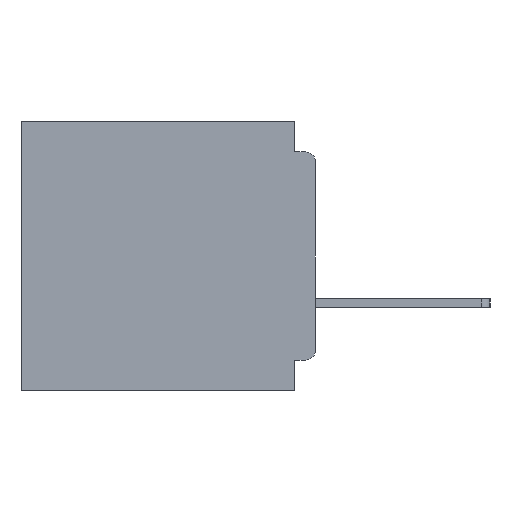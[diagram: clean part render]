
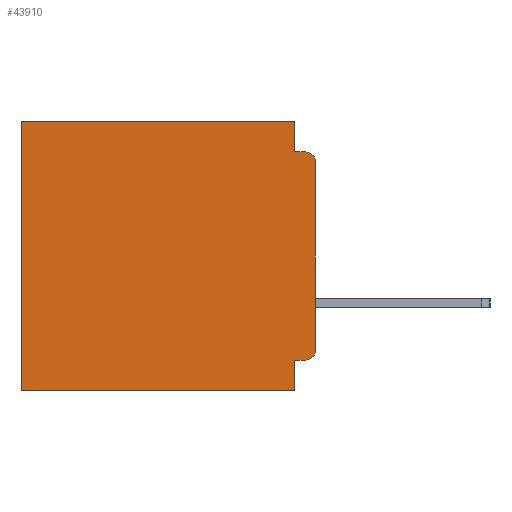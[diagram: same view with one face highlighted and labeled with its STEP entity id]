
A CAD part, left-side view. The second image highlights one B-rep face of the part: STEP entity #43910.
In plain terms, the highlighted planar face has unit normal (-1, 0, 0).
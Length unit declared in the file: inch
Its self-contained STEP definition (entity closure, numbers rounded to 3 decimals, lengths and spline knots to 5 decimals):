
#1791 = DIRECTION ( 'NONE',  ( -1., 0., 0. ) ) ;
#1885 = FACE_OUTER_BOUND ( 'NONE', #11397, .T. ) ;
#2329 = CARTESIAN_POINT ( 'NONE',  ( 0.3, 0., -0.355 ) ) ;
#4310 = EDGE_CURVE ( 'NONE', #43172, #33014, #31219, .T. ) ;
#4643 = LINE ( 'NONE', #56079, #29865 ) ;
#5881 = CARTESIAN_POINT ( 'NONE',  ( 0.3, 0.031, -0.4 ) ) ;
#5959 = ORIENTED_EDGE ( 'NONE', *, *, #39937, .F. ) ;
#6183 = EDGE_CURVE ( 'NONE', #24447, #8445, #24903, .T. ) ;
#6184 = DIRECTION ( 'NONE',  ( 0., 1., 0. ) ) ;
#6205 = ORIENTED_EDGE ( 'NONE', *, *, #42657, .F. ) ;
#7471 = EDGE_CURVE ( 'NONE', #31650, #18828, #55676, .T. ) ;
#8445 = VERTEX_POINT ( 'NONE', #22327 ) ;
#8450 = VECTOR ( 'NONE', #27297, 39.37008 ) ;
#10390 = DIRECTION ( 'NONE',  ( 0., 0., -1. ) ) ;
#11123 = EDGE_CURVE ( 'NONE', #57557, #18828, #26857, .T. ) ;
#11397 = EDGE_LOOP ( 'NONE', ( #47366, #43980, #29341, #6205, #17190, #47923, #54518, #5959, #53245, #41946 ) ) ;
#12520 = CARTESIAN_POINT ( 'NONE',  ( 0.3, 0., -0.4 ) ) ;
#15496 = CARTESIAN_POINT ( 'NONE',  ( 0.3, 0.015, -0.045 ) ) ;
#15551 = DIRECTION ( 'NONE',  ( 0., 0., -1. ) ) ;
#16003 = CARTESIAN_POINT ( 'NONE',  ( 0.3, 0.437, -0.4 ) ) ;
#16267 = LINE ( 'NONE', #5881, #38499 ) ;
#17190 = ORIENTED_EDGE ( 'NONE', *, *, #36540, .T. ) ;
#17398 = EDGE_CURVE ( 'NONE', #31650, #33014, #44601, .T. ) ;
#17759 = DIRECTION ( 'NONE',  ( 1., 0., 0. ) ) ;
#18029 = CARTESIAN_POINT ( 'NONE',  ( 0.3, 0., -0.045 ) ) ;
#18828 = VERTEX_POINT ( 'NONE', #15496 ) ;
#19538 = CARTESIAN_POINT ( 'NONE',  ( 0.3, 0., 0. ) ) ;
#20397 = LINE ( 'NONE', #22845, #8450 ) ;
#20860 = LINE ( 'NONE', #19538, #42989 ) ;
#22327 = CARTESIAN_POINT ( 'NONE',  ( 0.3, 0.437, -0.4 ) ) ;
#22496 = LINE ( 'NONE', #2329, #57568 ) ;
#22845 = CARTESIAN_POINT ( 'NONE',  ( 0.3, 0., -0.4 ) ) ;
#23494 = VECTOR ( 'NONE', #15551, 39.37008 ) ;
#23958 = EDGE_CURVE ( 'NONE', #43172, #37621, #22496, .T. ) ;
#24447 = VERTEX_POINT ( 'NONE', #45689 ) ;
#24903 = LINE ( 'NONE', #16003, #23494 ) ;
#25475 = VECTOR ( 'NONE', #48990, 39.37008 ) ;
#25544 = CARTESIAN_POINT ( 'NONE',  ( 0.3, 0.031, 0. ) ) ;
#26857 = LINE ( 'NONE', #18029, #25475 ) ;
#27297 = DIRECTION ( 'NONE',  ( 0., 1., 0. ) ) ;
#28343 = CARTESIAN_POINT ( 'NONE',  ( 0.3, 0.031, -0.4 ) ) ;
#28641 = CARTESIAN_POINT ( 'NONE',  ( 0.3, 0.015, -0.06 ) ) ;
#29341 = ORIENTED_EDGE ( 'NONE', *, *, #11123, .F. ) ;
#29607 = VERTEX_POINT ( 'NONE', #28343 ) ;
#29787 = DIRECTION ( 'NONE',  ( 0., 0., -1. ) ) ;
#29865 = VECTOR ( 'NONE', #29787, 39.37008 ) ;
#31219 = CIRCLE ( 'NONE', #49238, 0.015 ) ;
#31650 = VERTEX_POINT ( 'NONE', #43551 ) ;
#33014 = VERTEX_POINT ( 'NONE', #45607 ) ;
#33081 = DIRECTION ( 'NONE',  ( 0., 0., -1. ) ) ;
#33795 = DIRECTION ( 'NONE',  ( 0., 1., 0. ) ) ;
#34643 = EDGE_CURVE ( 'NONE', #29607, #8445, #20397, .T. ) ;
#36540 = EDGE_CURVE ( 'NONE', #40881, #24447, #20860, .T. ) ;
#37621 = VERTEX_POINT ( 'NONE', #45113 ) ;
#38499 = VECTOR ( 'NONE', #10390, 39.37008 ) ;
#39677 = PLANE ( 'NONE',  #48387 ) ;
#39937 = EDGE_CURVE ( 'NONE', #37621, #29607, #16267, .T. ) ;
#40881 = VERTEX_POINT ( 'NONE', #25544 ) ;
#41946 = ORIENTED_EDGE ( 'NONE', *, *, #4310, .T. ) ;
#42657 = EDGE_CURVE ( 'NONE', #40881, #57557, #4643, .T. ) ;
#42989 = VECTOR ( 'NONE', #6184, 39.37008 ) ;
#43172 = VERTEX_POINT ( 'NONE', #50726 ) ;
#43551 = CARTESIAN_POINT ( 'NONE',  ( 0.3, 0., -0.06 ) ) ;
#43910 = ADVANCED_FACE ( 'NONE', ( #1885 ), #39677, .F. ) ;
#43980 = ORIENTED_EDGE ( 'NONE', *, *, #7471, .T. ) ;
#44282 = CARTESIAN_POINT ( 'NONE',  ( 0.3, 0., -0.4 ) ) ;
#44601 = LINE ( 'NONE', #12520, #54872 ) ;
#45113 = CARTESIAN_POINT ( 'NONE',  ( 0.3, 0.031, -0.355 ) ) ;
#45607 = CARTESIAN_POINT ( 'NONE',  ( 0.3, 0., -0.34 ) ) ;
#45689 = CARTESIAN_POINT ( 'NONE',  ( 0.3, 0.437, 0. ) ) ;
#46176 = CARTESIAN_POINT ( 'NONE',  ( 0.3, 0.031, -0.045 ) ) ;
#47366 = ORIENTED_EDGE ( 'NONE', *, *, #17398, .F. ) ;
#47923 = ORIENTED_EDGE ( 'NONE', *, *, #6183, .T. ) ;
#48387 = AXIS2_PLACEMENT_3D ( 'NONE', #44282, #17759, #48720 ) ;
#48720 = DIRECTION ( 'NONE',  ( 0., 0., -1. ) ) ;
#48990 = DIRECTION ( 'NONE',  ( 0., -1., 0. ) ) ;
#49238 = AXIS2_PLACEMENT_3D ( 'NONE', #54701, #54526, #52601 ) ;
#50726 = CARTESIAN_POINT ( 'NONE',  ( 0.3, 0.015, -0.355 ) ) ;
#52601 = DIRECTION ( 'NONE',  ( 0., 0., -1. ) ) ;
#53245 = ORIENTED_EDGE ( 'NONE', *, *, #23958, .F. ) ;
#54518 = ORIENTED_EDGE ( 'NONE', *, *, #34643, .F. ) ;
#54526 = DIRECTION ( 'NONE',  ( -1., 0., 0. ) ) ;
#54701 = CARTESIAN_POINT ( 'NONE',  ( 0.3, 0.015, -0.34 ) ) ;
#54872 = VECTOR ( 'NONE', #56579, 39.37008 ) ;
#55578 = AXIS2_PLACEMENT_3D ( 'NONE', #28641, #1791, #33081 ) ;
#55676 = CIRCLE ( 'NONE', #55578, 0.015 ) ;
#56079 = CARTESIAN_POINT ( 'NONE',  ( 0.3, 0.031, 0. ) ) ;
#56579 = DIRECTION ( 'NONE',  ( 0., 0., -1. ) ) ;
#57557 = VERTEX_POINT ( 'NONE', #46176 ) ;
#57568 = VECTOR ( 'NONE', #33795, 39.37008 ) ;
